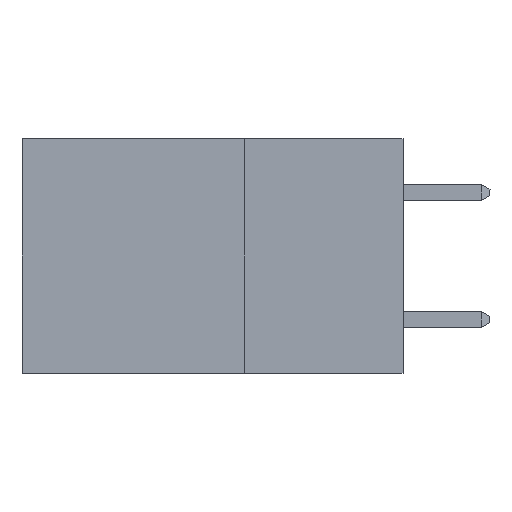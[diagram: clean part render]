
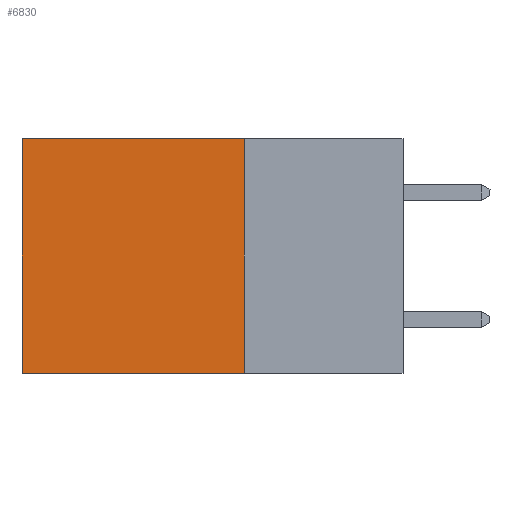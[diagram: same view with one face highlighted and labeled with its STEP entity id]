
A CAD part, left-side view. The second image highlights one B-rep face of the part: STEP entity #6830.
In plain terms, the highlighted planar face has unit normal (-1, 0, 0).
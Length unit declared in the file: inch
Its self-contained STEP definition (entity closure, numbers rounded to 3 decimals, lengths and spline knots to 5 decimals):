
#692 = ORIENTED_EDGE ( 'NONE', *, *, #2231, .F. ) ;
#809 = LINE ( 'NONE', #8685, #10799 ) ;
#1320 = FACE_OUTER_BOUND ( 'NONE', #11428, .T. ) ;
#1713 = CARTESIAN_POINT ( 'NONE',  ( 0.2875, 0.25, 0. ) ) ;
#1824 = AXIS2_PLACEMENT_3D ( 'NONE', #1713, #11588, #5793 ) ;
#1882 = EDGE_CURVE ( 'NONE', #9992, #11042, #11504, .T. ) ;
#1976 = EDGE_CURVE ( 'NONE', #11042, #10853, #3093, .T. ) ;
#2231 = EDGE_CURVE ( 'NONE', #9401, #10853, #809, .T. ) ;
#2788 = LINE ( 'NONE', #9983, #12510 ) ;
#3093 = LINE ( 'NONE', #10087, #8131 ) ;
#5207 = CARTESIAN_POINT ( 'NONE',  ( 0.2875, 0.25, 0. ) ) ;
#5277 = CARTESIAN_POINT ( 'NONE',  ( 0.2875, 0.6, -0.37 ) ) ;
#5793 = DIRECTION ( 'NONE',  ( 0., 0., -1. ) ) ;
#6116 = ORIENTED_EDGE ( 'NONE', *, *, #12696, .F. ) ;
#6830 = ADVANCED_FACE ( 'NONE', ( #1320 ), #8786, .F. ) ;
#8131 = VECTOR ( 'NONE', #10143, 39.37008 ) ;
#8465 = ORIENTED_EDGE ( 'NONE', *, *, #1976, .T. ) ;
#8685 = CARTESIAN_POINT ( 'NONE',  ( 0.2875, 0.25, -0.37 ) ) ;
#8712 = DIRECTION ( 'NONE',  ( 0., 1., 0. ) ) ;
#8786 = PLANE ( 'NONE',  #1824 ) ;
#9401 = VERTEX_POINT ( 'NONE', #12123 ) ;
#9983 = CARTESIAN_POINT ( 'NONE',  ( 0.2875, 0.25, 0. ) ) ;
#9992 = VERTEX_POINT ( 'NONE', #5207 ) ;
#10087 = CARTESIAN_POINT ( 'NONE',  ( 0.2875, 0.6, 0. ) ) ;
#10143 = DIRECTION ( 'NONE',  ( 0., 0., -1. ) ) ;
#10459 = DIRECTION ( 'NONE',  ( 0., 1., 0. ) ) ;
#10673 = CARTESIAN_POINT ( 'NONE',  ( 0.2875, 0.25, 0. ) ) ;
#10799 = VECTOR ( 'NONE', #8712, 39.37008 ) ;
#10853 = VERTEX_POINT ( 'NONE', #5277 ) ;
#10950 = DIRECTION ( 'NONE',  ( 0., 0., -1. ) ) ;
#11042 = VERTEX_POINT ( 'NONE', #12175 ) ;
#11221 = VECTOR ( 'NONE', #10459, 39.37008 ) ;
#11428 = EDGE_LOOP ( 'NONE', ( #8465, #692, #6116, #11532 ) ) ;
#11504 = LINE ( 'NONE', #10673, #11221 ) ;
#11532 = ORIENTED_EDGE ( 'NONE', *, *, #1882, .T. ) ;
#11588 = DIRECTION ( 'NONE',  ( 1., 0., 0. ) ) ;
#12123 = CARTESIAN_POINT ( 'NONE',  ( 0.2875, 0.25, -0.37 ) ) ;
#12175 = CARTESIAN_POINT ( 'NONE',  ( 0.2875, 0.6, 0. ) ) ;
#12510 = VECTOR ( 'NONE', #10950, 39.37008 ) ;
#12696 = EDGE_CURVE ( 'NONE', #9992, #9401, #2788, .T. ) ;
